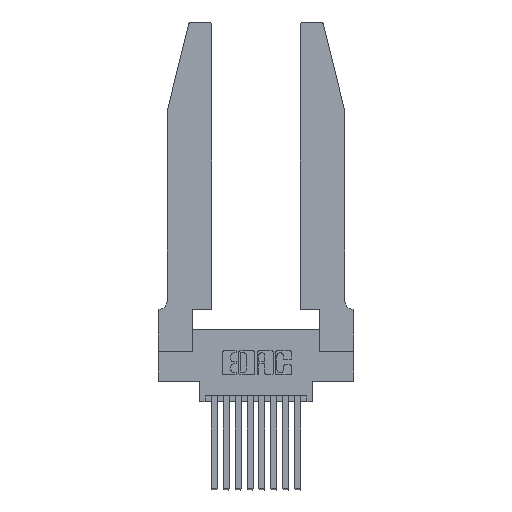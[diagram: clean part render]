
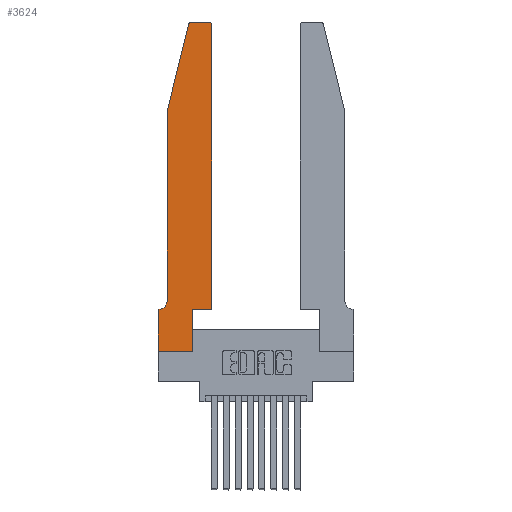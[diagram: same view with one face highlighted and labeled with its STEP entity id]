
A CAD part, top view. The second image highlights one B-rep face of the part: STEP entity #3624.
In plain terms, the highlighted planar face has unit normal (0, 0, 1).
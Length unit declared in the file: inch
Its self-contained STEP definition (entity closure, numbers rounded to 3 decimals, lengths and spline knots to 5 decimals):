
#9 = FACE_OUTER_BOUND ( 'NONE', #1494, .T. ) ;
#447 = LINE ( 'NONE', #9826, #3483 ) ;
#902 = ORIENTED_EDGE ( 'NONE', *, *, #4793, .T. ) ;
#920 = VECTOR ( 'NONE', #5462, 39.37008 ) ;
#1011 = VERTEX_POINT ( 'NONE', #2050 ) ;
#1151 = DIRECTION ( 'NONE',  ( 1., 0., 0. ) ) ;
#1153 = DIRECTION ( 'NONE',  ( 0., 0., 1. ) ) ;
#1174 = CARTESIAN_POINT ( 'NONE',  ( 0.4205, 2.72, 0.37 ) ) ;
#1494 = EDGE_LOOP ( 'NONE', ( #15168, #11521, #10581, #4607, #902, #14869, #6388, #9637, #2516, #4120, #6748, #11961 ) ) ;
#2029 = LINE ( 'NONE', #14768, #8581 ) ;
#2050 = CARTESIAN_POINT ( 'NONE',  ( 0.2865, 0., 0.37 ) ) ;
#2402 = VECTOR ( 'NONE', #9229, 39.37008 ) ;
#2435 = VECTOR ( 'NONE', #12232, 39.37008 ) ;
#2463 = CARTESIAN_POINT ( 'NONE',  ( 0.0055, 0.35, 0.37 ) ) ;
#2516 = ORIENTED_EDGE ( 'NONE', *, *, #7014, .T. ) ;
#2605 = DIRECTION ( 'NONE',  ( 0., 0., 1. ) ) ;
#2811 = LINE ( 'NONE', #8022, #2402 ) ;
#3409 = VERTEX_POINT ( 'NONE', #13004 ) ;
#3427 = AXIS2_PLACEMENT_3D ( 'NONE', #12651, #5640, #13801 ) ;
#3483 = VECTOR ( 'NONE', #3872, 39.37008 ) ;
#3624 = ADVANCED_FACE ( 'NONE', ( #9 ), #5056, .T. ) ;
#3707 = EDGE_CURVE ( 'NONE', #3740, #11276, #14528, .T. ) ;
#3740 = VERTEX_POINT ( 'NONE', #2463 ) ;
#3853 = EDGE_CURVE ( 'NONE', #7872, #11424, #7286, .T. ) ;
#3872 = DIRECTION ( 'NONE',  ( 1., 0., 0. ) ) ;
#4120 = ORIENTED_EDGE ( 'NONE', *, *, #7059, .T. ) ;
#4200 = CARTESIAN_POINT ( 'NONE',  ( 0.0755, 2., 0.37 ) ) ;
#4465 = CARTESIAN_POINT ( 'NONE',  ( 0.0755, 0.35, 0.37 ) ) ;
#4518 = DIRECTION ( 'NONE',  ( 1., 0., 0. ) ) ;
#4607 = ORIENTED_EDGE ( 'NONE', *, *, #11007, .T. ) ;
#4793 = EDGE_CURVE ( 'NONE', #7082, #3740, #12205, .T. ) ;
#4827 = CARTESIAN_POINT ( 'NONE',  ( 0., 0.35, 0.37 ) ) ;
#4885 = CARTESIAN_POINT ( 'NONE',  ( 0.2605, 2.75, 0.37 ) ) ;
#4900 = EDGE_CURVE ( 'NONE', #8406, #10263, #14151, .T. ) ;
#5056 = PLANE ( 'NONE',  #12881 ) ;
#5439 = DIRECTION ( 'NONE',  ( 0., 0., -1. ) ) ;
#5462 = DIRECTION ( 'NONE',  ( 0., -1., 0. ) ) ;
#5640 = DIRECTION ( 'NONE',  ( 0., 0., 1. ) ) ;
#6196 = DIRECTION ( 'NONE',  ( -1., 0., 0. ) ) ;
#6219 = DIRECTION ( 'NONE',  ( 0., 1., 0. ) ) ;
#6359 = AXIS2_PLACEMENT_3D ( 'NONE', #1174, #1153, #1151 ) ;
#6388 = ORIENTED_EDGE ( 'NONE', *, *, #14298, .T. ) ;
#6510 = CARTESIAN_POINT ( 'NONE',  ( 0.4205, 2.75, 0.37 ) ) ;
#6748 = ORIENTED_EDGE ( 'NONE', *, *, #8343, .T. ) ;
#6769 = VERTEX_POINT ( 'NONE', #12785 ) ;
#7014 = EDGE_CURVE ( 'NONE', #1011, #9713, #10635, .T. ) ;
#7043 = CARTESIAN_POINT ( 'NONE',  ( 0.4505, 0.35, 0.37 ) ) ;
#7059 = EDGE_CURVE ( 'NONE', #9713, #9965, #447, .T. ) ;
#7082 = VERTEX_POINT ( 'NONE', #12201 ) ;
#7286 = CIRCLE ( 'NONE', #6359, 0.03 ) ;
#7524 = EDGE_CURVE ( 'NONE', #10263, #3409, #10266, .T. ) ;
#7872 = VERTEX_POINT ( 'NONE', #10374 ) ;
#8022 = CARTESIAN_POINT ( 'NONE',  ( 0., 0., 0.37 ) ) ;
#8270 = CARTESIAN_POINT ( 'NONE',  ( 0.2865, 0.35, 0.37 ) ) ;
#8343 = EDGE_CURVE ( 'NONE', #9965, #7872, #2029, .T. ) ;
#8406 = VERTEX_POINT ( 'NONE', #10267 ) ;
#8463 = CARTESIAN_POINT ( 'NONE',  ( 0., 0.35, 0.37 ) ) ;
#8581 = VECTOR ( 'NONE', #12482, 39.37008 ) ;
#8817 = EDGE_CURVE ( 'NONE', #6769, #1011, #12732, .T. ) ;
#9229 = DIRECTION ( 'NONE',  ( 0., -1., 0. ) ) ;
#9637 = ORIENTED_EDGE ( 'NONE', *, *, #8817, .T. ) ;
#9713 = VERTEX_POINT ( 'NONE', #8270 ) ;
#9826 = CARTESIAN_POINT ( 'NONE',  ( 0.4505, 0.35, 0.37 ) ) ;
#9965 = VERTEX_POINT ( 'NONE', #7043 ) ;
#10263 = VERTEX_POINT ( 'NONE', #13505 ) ;
#10266 = LINE ( 'NONE', #12008, #12953 ) ;
#10267 = CARTESIAN_POINT ( 'NONE',  ( 0.284, 2.75, 0.37 ) ) ;
#10335 = LINE ( 'NONE', #4200, #920 ) ;
#10374 = CARTESIAN_POINT ( 'NONE',  ( 0.4505, 2.72, 0.37 ) ) ;
#10581 = ORIENTED_EDGE ( 'NONE', *, *, #7524, .T. ) ;
#10635 = LINE ( 'NONE', #14325, #13701 ) ;
#11007 = EDGE_CURVE ( 'NONE', #3409, #7082, #10335, .T. ) ;
#11075 = CARTESIAN_POINT ( 'NONE',  ( 0., 0., 0.37 ) ) ;
#11276 = VERTEX_POINT ( 'NONE', #8463 ) ;
#11424 = VERTEX_POINT ( 'NONE', #6510 ) ;
#11487 = VECTOR ( 'NONE', #6196, 39.37008 ) ;
#11521 = ORIENTED_EDGE ( 'NONE', *, *, #4900, .T. ) ;
#11804 = EDGE_CURVE ( 'NONE', #11424, #8406, #12126, .T. ) ;
#11961 = ORIENTED_EDGE ( 'NONE', *, *, #3853, .T. ) ;
#12008 = CARTESIAN_POINT ( 'NONE',  ( 0.0755, 2., 0.37 ) ) ;
#12126 = LINE ( 'NONE', #4885, #15129 ) ;
#12201 = CARTESIAN_POINT ( 'NONE',  ( 0.0755, 0.42, 0.37 ) ) ;
#12205 = CIRCLE ( 'NONE', #13303, 0.07 ) ;
#12232 = DIRECTION ( 'NONE',  ( 1., 0., 0. ) ) ;
#12462 = CARTESIAN_POINT ( 'NONE',  ( 0.0055, 0.42, 0.37 ) ) ;
#12482 = DIRECTION ( 'NONE',  ( 0., 1., 0. ) ) ;
#12651 = CARTESIAN_POINT ( 'NONE',  ( 0.284, 2.72, 0.37 ) ) ;
#12732 = LINE ( 'NONE', #11075, #2435 ) ;
#12785 = CARTESIAN_POINT ( 'NONE',  ( 0., 0., 0.37 ) ) ;
#12881 = AXIS2_PLACEMENT_3D ( 'NONE', #4827, #2605, #4518 ) ;
#12953 = VECTOR ( 'NONE', #13168, 39.37008 ) ;
#13004 = CARTESIAN_POINT ( 'NONE',  ( 0.0755, 2., 0.37 ) ) ;
#13113 = DIRECTION ( 'NONE',  ( -1., 0., 0. ) ) ;
#13168 = DIRECTION ( 'NONE',  ( -0.239, -0.971, 0. ) ) ;
#13303 = AXIS2_PLACEMENT_3D ( 'NONE', #12462, #5439, #13619 ) ;
#13505 = CARTESIAN_POINT ( 'NONE',  ( 0.25487, 2.72718, 0.37 ) ) ;
#13619 = DIRECTION ( 'NONE',  ( -1., 0., 0. ) ) ;
#13701 = VECTOR ( 'NONE', #6219, 39.37008 ) ;
#13801 = DIRECTION ( 'NONE',  ( 1., 0., 0. ) ) ;
#14151 = CIRCLE ( 'NONE', #3427, 0.03 ) ;
#14298 = EDGE_CURVE ( 'NONE', #11276, #6769, #2811, .T. ) ;
#14325 = CARTESIAN_POINT ( 'NONE',  ( 0.2865, 0.35, 0.37 ) ) ;
#14528 = LINE ( 'NONE', #4465, #11487 ) ;
#14768 = CARTESIAN_POINT ( 'NONE',  ( 0.4505, 0.35, 0.37 ) ) ;
#14869 = ORIENTED_EDGE ( 'NONE', *, *, #3707, .T. ) ;
#15129 = VECTOR ( 'NONE', #13113, 39.37008 ) ;
#15168 = ORIENTED_EDGE ( 'NONE', *, *, #11804, .T. ) ;
